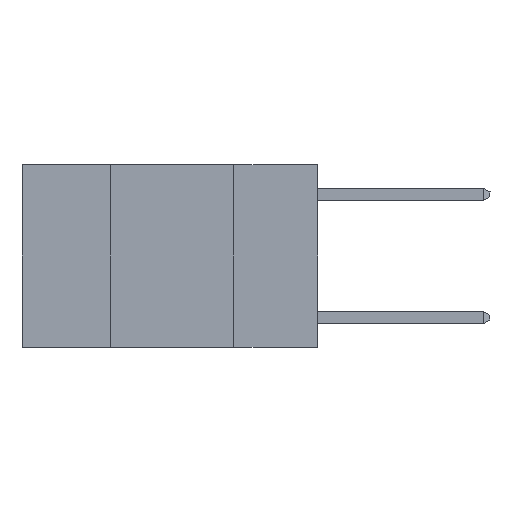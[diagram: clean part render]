
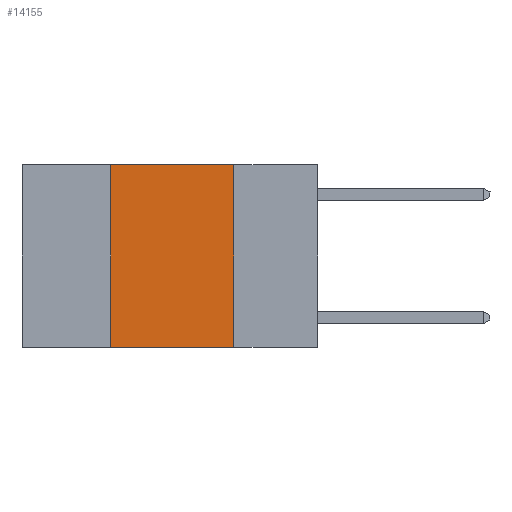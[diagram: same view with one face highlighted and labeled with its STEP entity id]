
A CAD part, left-side view. The second image highlights one B-rep face of the part: STEP entity #14155.
In plain terms, the highlighted planar face has unit normal (-1, 0, 0).
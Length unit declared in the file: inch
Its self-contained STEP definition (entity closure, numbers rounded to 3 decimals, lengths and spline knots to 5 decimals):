
#723 = LINE ( 'NONE', #1142, #10894 ) ;
#846 = VECTOR ( 'NONE', #8092, 39.37008 ) ;
#1142 = CARTESIAN_POINT ( 'NONE',  ( 0., 0.17, 0. ) ) ;
#2296 = CARTESIAN_POINT ( 'NONE',  ( 0., 0.42, 0. ) ) ;
#2688 = DIRECTION ( 'NONE',  ( 0., 0., -1. ) ) ;
#3038 = EDGE_CURVE ( 'NONE', #16803, #17910, #4204, .T. ) ;
#4007 = DIRECTION ( 'NONE',  ( 0., 0., -1. ) ) ;
#4204 = LINE ( 'NONE', #11334, #9759 ) ;
#4558 = CARTESIAN_POINT ( 'NONE',  ( 0., 0.6, 0. ) ) ;
#6331 = VERTEX_POINT ( 'NONE', #2296 ) ;
#7694 = DIRECTION ( 'NONE',  ( 1., 0., 0. ) ) ;
#7998 = LINE ( 'NONE', #4558, #21179 ) ;
#8092 = DIRECTION ( 'NONE',  ( 0., 0., 1. ) ) ;
#8216 = EDGE_CURVE ( 'NONE', #6331, #9307, #7998, .T. ) ;
#8218 = ORIENTED_EDGE ( 'NONE', *, *, #15817, .F. ) ;
#8844 = CARTESIAN_POINT ( 'NONE',  ( 0., 0.17, 0. ) ) ;
#9035 = ORIENTED_EDGE ( 'NONE', *, *, #3038, .T. ) ;
#9307 = VERTEX_POINT ( 'NONE', #8844 ) ;
#9759 = VECTOR ( 'NONE', #11539, 39.37008 ) ;
#9838 = EDGE_CURVE ( 'NONE', #16803, #6331, #16279, .T. ) ;
#9964 = ORIENTED_EDGE ( 'NONE', *, *, #8216, .F. ) ;
#10894 = VECTOR ( 'NONE', #4007, 39.37008 ) ;
#11047 = FACE_OUTER_BOUND ( 'NONE', #13609, .T. ) ;
#11334 = CARTESIAN_POINT ( 'NONE',  ( 0., 0.6, -0.37 ) ) ;
#11539 = DIRECTION ( 'NONE',  ( 0., -1., 0. ) ) ;
#12660 = AXIS2_PLACEMENT_3D ( 'NONE', #17829, #7694, #2688 ) ;
#13609 = EDGE_LOOP ( 'NONE', ( #8218, #9964, #19254, #9035 ) ) ;
#14155 = ADVANCED_FACE ( 'NONE', ( #11047 ), #17731, .F. ) ;
#15604 = CARTESIAN_POINT ( 'NONE',  ( 0., 0.17, -0.37 ) ) ;
#15817 = EDGE_CURVE ( 'NONE', #9307, #17910, #723, .T. ) ;
#16253 = CARTESIAN_POINT ( 'NONE',  ( 0., 0.42, -0.37 ) ) ;
#16279 = LINE ( 'NONE', #20920, #846 ) ;
#16803 = VERTEX_POINT ( 'NONE', #16253 ) ;
#17731 = PLANE ( 'NONE',  #12660 ) ;
#17829 = CARTESIAN_POINT ( 'NONE',  ( 0., 0.6, 0. ) ) ;
#17910 = VERTEX_POINT ( 'NONE', #15604 ) ;
#19254 = ORIENTED_EDGE ( 'NONE', *, *, #9838, .F. ) ;
#20920 = CARTESIAN_POINT ( 'NONE',  ( 0., 0.42, 0. ) ) ;
#21179 = VECTOR ( 'NONE', #21554, 39.37008 ) ;
#21554 = DIRECTION ( 'NONE',  ( 0., -1., 0. ) ) ;
